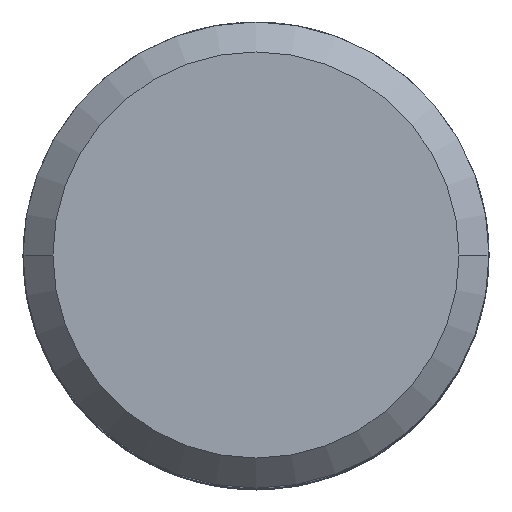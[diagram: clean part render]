
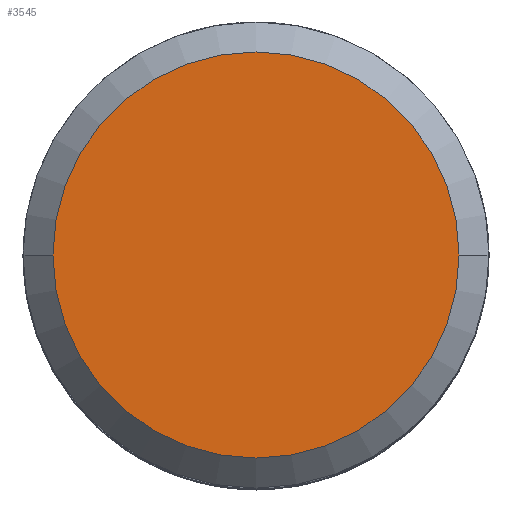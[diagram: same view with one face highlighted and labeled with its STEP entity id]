
A CAD part, top view. The second image highlights one B-rep face of the part: STEP entity #3545.
In plain terms, the highlighted planar face has unit normal (0, 0, 1).
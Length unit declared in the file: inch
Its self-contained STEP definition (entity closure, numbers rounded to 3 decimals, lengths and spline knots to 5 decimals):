
#543=CARTESIAN_POINT('',(0.,0.,0.93));
#544=DIRECTION('',(0.,0.,1.));
#545=DIRECTION('',(1.,0.,0.));
#546=AXIS2_PLACEMENT_3D('',#543,#544,#545);
#551=CARTESIAN_POINT('',(0.,0.,0.93));
#552=DIRECTION('',(0.,0.,1.));
#553=DIRECTION('',(-1.,0.,0.));
#554=AXIS2_PLACEMENT_3D('',#551,#552,#553);
#3143=CARTESIAN_POINT('',(0.1625,0.,0.93));
#3145=VERTEX_POINT('',#3143);
#3147=CARTESIAN_POINT('',(-0.1625,0.,0.93));
#3149=VERTEX_POINT('',#3147);
#3536=CARTESIAN_POINT('',(0.,0.,0.93));
#3537=DIRECTION('',(0.,0.,1.));
#3538=DIRECTION('',(1.,0.,0.));
#3539=AXIS2_PLACEMENT_3D('',#3536,#3537,#3538);
#3540=PLANE('',#3539);
#3541=ORIENTED_EDGE('',*,*,#3530,.F.);
#3542=ORIENTED_EDGE('',*,*,#3516,.F.);
#3543=EDGE_LOOP('',(#3541,#3542));
#3544=FACE_OUTER_BOUND('',#3543,.F.);
#547=CIRCLE('',#546,0.1625);
#555=CIRCLE('',#554,0.1625);
#3516=EDGE_CURVE('',#3149,#3145,#555,.T.);
#3530=EDGE_CURVE('',#3145,#3149,#547,.T.);
#3545=ADVANCED_FACE('',(#3544),#3540,.T.);
